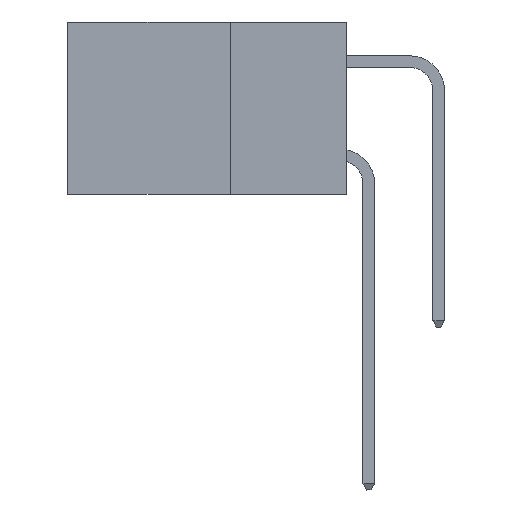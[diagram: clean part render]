
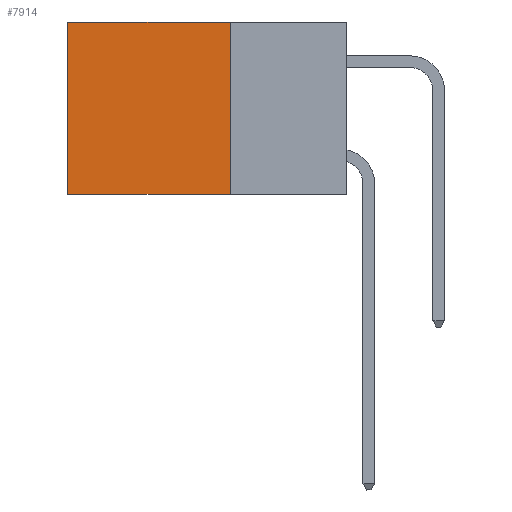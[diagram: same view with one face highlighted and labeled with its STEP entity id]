
A CAD part, left-side view. The second image highlights one B-rep face of the part: STEP entity #7914.
In plain terms, the highlighted planar face has unit normal (-1, 0, 0).
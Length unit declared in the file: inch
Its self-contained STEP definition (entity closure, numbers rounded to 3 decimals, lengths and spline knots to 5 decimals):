
#337 = EDGE_CURVE ( 'NONE', #2069, #3685, #12151, .T. ) ;
#1397 = CARTESIAN_POINT ( 'NONE',  ( 0.2875, 0.6, 0. ) ) ;
#1804 = EDGE_CURVE ( 'NONE', #3074, #10690, #9910, .T. ) ;
#2069 = VERTEX_POINT ( 'NONE', #1397 ) ;
#2076 = CARTESIAN_POINT ( 'NONE',  ( 0.2875, 0.25, -0.37 ) ) ;
#3074 = VERTEX_POINT ( 'NONE', #10896 ) ;
#3317 = VECTOR ( 'NONE', #9159, 39.37008 ) ;
#3685 = VERTEX_POINT ( 'NONE', #8814 ) ;
#3723 = PLANE ( 'NONE',  #8365 ) ;
#4227 = VECTOR ( 'NONE', #10837, 39.37008 ) ;
#4535 = VECTOR ( 'NONE', #9234, 39.37008 ) ;
#4679 = ORIENTED_EDGE ( 'NONE', *, *, #6795, .T. ) ;
#5030 = EDGE_CURVE ( 'NONE', #10690, #3685, #5214, .T. ) ;
#5214 = LINE ( 'NONE', #2076, #12700 ) ;
#5874 = DIRECTION ( 'NONE',  ( 1., 0., 0. ) ) ;
#6136 = LINE ( 'NONE', #10106, #3317 ) ;
#6229 = DIRECTION ( 'NONE',  ( 0., 1., 0. ) ) ;
#6740 = CARTESIAN_POINT ( 'NONE',  ( 0.2875, 0.25, -0.37 ) ) ;
#6759 = ORIENTED_EDGE ( 'NONE', *, *, #337, .T. ) ;
#6795 = EDGE_CURVE ( 'NONE', #3074, #2069, #6136, .T. ) ;
#7080 = ORIENTED_EDGE ( 'NONE', *, *, #1804, .F. ) ;
#7853 = CARTESIAN_POINT ( 'NONE',  ( 0.2875, 0.25, 0. ) ) ;
#7914 = ADVANCED_FACE ( 'NONE', ( #11184 ), #3723, .F. ) ;
#8365 = AXIS2_PLACEMENT_3D ( 'NONE', #7853, #5874, #12660 ) ;
#8814 = CARTESIAN_POINT ( 'NONE',  ( 0.2875, 0.6, -0.37 ) ) ;
#9159 = DIRECTION ( 'NONE',  ( 0., 1., 0. ) ) ;
#9234 = DIRECTION ( 'NONE',  ( 0., 0., -1. ) ) ;
#9910 = LINE ( 'NONE', #12962, #4535 ) ;
#10106 = CARTESIAN_POINT ( 'NONE',  ( 0.2875, 0.25, 0. ) ) ;
#10677 = EDGE_LOOP ( 'NONE', ( #6759, #11953, #7080, #4679 ) ) ;
#10690 = VERTEX_POINT ( 'NONE', #6740 ) ;
#10771 = CARTESIAN_POINT ( 'NONE',  ( 0.2875, 0.6, 0. ) ) ;
#10837 = DIRECTION ( 'NONE',  ( 0., 0., -1. ) ) ;
#10896 = CARTESIAN_POINT ( 'NONE',  ( 0.2875, 0.25, 0. ) ) ;
#11184 = FACE_OUTER_BOUND ( 'NONE', #10677, .T. ) ;
#11953 = ORIENTED_EDGE ( 'NONE', *, *, #5030, .F. ) ;
#12151 = LINE ( 'NONE', #10771, #4227 ) ;
#12660 = DIRECTION ( 'NONE',  ( 0., 0., -1. ) ) ;
#12700 = VECTOR ( 'NONE', #6229, 39.37008 ) ;
#12962 = CARTESIAN_POINT ( 'NONE',  ( 0.2875, 0.25, 0. ) ) ;
